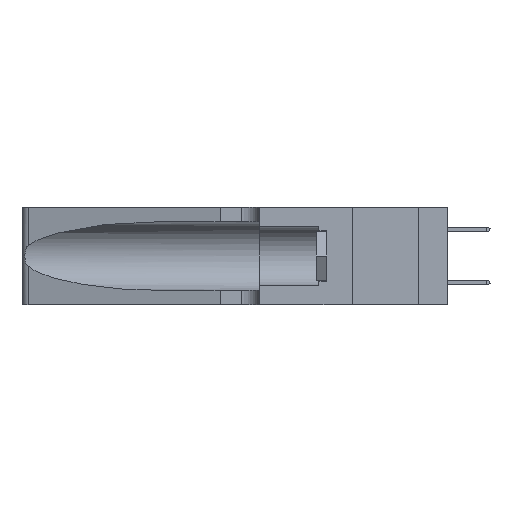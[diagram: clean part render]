
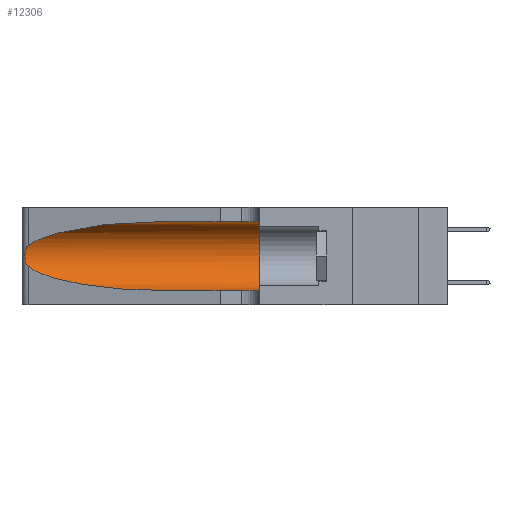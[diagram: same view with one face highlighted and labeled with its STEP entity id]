
A CAD part, left-side view. The second image highlights one B-rep face of the part: STEP entity #12306.
In plain terms, the highlighted cylindrical face has radius 3.308 mm (diameter 6.617 mm), a partial arc.
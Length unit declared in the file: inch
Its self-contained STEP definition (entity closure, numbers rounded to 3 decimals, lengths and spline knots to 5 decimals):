
#554 = CARTESIAN_POINT ( 'NONE',  ( 0.1305, 0.72297, 0.05475 ) ) ;
#833 =( BOUNDED_CURVE ( )  B_SPLINE_CURVE ( 3, ( #21666, #19783, #14229, #2589 ),
 .UNSPECIFIED., .F., .F. ) 
 B_SPLINE_CURVE_WITH_KNOTS ( ( 4, 4 ),
 ( 1.5708, 2.84003 ),
 .UNSPECIFIED. ) 
 CURVE ( )  GEOMETRIC_REPRESENTATION_ITEM ( )  RATIONAL_B_SPLINE_CURVE ( ( 1., 0.87, 0.87, 1. ) ) 
 REPRESENTATION_ITEM ( '' )  );
#1058 = CARTESIAN_POINT ( 'NONE',  ( 0.26075, 1.23896, 0.19203 ) ) ;
#1847 = CIRCLE ( 'NONE', #7283, 0.13025 ) ;
#2323 = VERTEX_POINT ( 'NONE', #22062 ) ;
#2327 = DIRECTION ( 'NONE',  ( 0., 1., 0. ) ) ;
#2589 = CARTESIAN_POINT ( 'NONE',  ( 0.25487, 1.22718, 0.22369 ) ) ;
#3119 = CARTESIAN_POINT ( 'NONE',  ( 0.26017, 1.23833, 0.17102 ) ) ;
#3168 = VERTEX_POINT ( 'NONE', #9739 ) ;
#3367 = ORIENTED_EDGE ( 'NONE', *, *, #22106, .T. ) ;
#3416 = CARTESIAN_POINT ( 'NONE',  ( 0.18966, 0.96281, 0.05475 ) ) ;
#4304 = ORIENTED_EDGE ( 'NONE', *, *, #17863, .F. ) ;
#4429 = CYLINDRICAL_SURFACE ( 'NONE', #19527, 0.13025 ) ;
#4578 =( BOUNDED_CURVE ( )  B_SPLINE_CURVE ( 3, ( #13120, #24311, #3416, #16892 ),
 .UNSPECIFIED., .F., .F. ) 
 B_SPLINE_CURVE_WITH_KNOTS ( ( 4, 4 ),
 ( 3.44316, 4.71239 ),
 .UNSPECIFIED. ) 
 CURVE ( )  GEOMETRIC_REPRESENTATION_ITEM ( )  RATIONAL_B_SPLINE_CURVE ( ( 1., 0.87, 0.87, 1. ) ) 
 REPRESENTATION_ITEM ( '' )  );
#4581 = B_SPLINE_CURVE_WITH_KNOTS ( 'NONE', 3,
 ( #12762, #9028, #22150, #10945, #24037, #12842, #1058, #14730, #3119, #16616, #5151, #18475, #7165, #20344 ),
 .UNSPECIFIED., .F., .F.,
 ( 4, 2, 2, 2, 2, 2, 4 ),
 ( 0., 0.00027, 0.00053, 0.00107, 0.0016, 0.00187, 0.00214 ),
 .UNSPECIFIED. ) ;
#5151 = CARTESIAN_POINT ( 'NONE',  ( 0.25789, 1.23486, 0.15765 ) ) ;
#6310 = EDGE_CURVE ( 'NONE', #8573, #9036, #4581, .T. ) ;
#7165 = CARTESIAN_POINT ( 'NONE',  ( 0.25555, 1.22993, 0.14849 ) ) ;
#7283 = AXIS2_PLACEMENT_3D ( 'NONE', #13997, #2327, #15899 ) ;
#8015 = CARTESIAN_POINT ( 'NONE',  ( 0.25487, 1.22718, 0.14631 ) ) ;
#8573 = VERTEX_POINT ( 'NONE', #17609 ) ;
#8667 = ORIENTED_EDGE ( 'NONE', *, *, #20192, .T. ) ;
#9028 = CARTESIAN_POINT ( 'NONE',  ( 0.25555, 1.22994, 0.2215 ) ) ;
#9036 = VERTEX_POINT ( 'NONE', #8015 ) ;
#9594 = EDGE_CURVE ( 'NONE', #23305, #2323, #19759, .T. ) ;
#9669 = FACE_OUTER_BOUND ( 'NONE', #20645, .T. ) ;
#9739 = CARTESIAN_POINT ( 'NONE',  ( 0.1305, 0.35, 0.05475 ) ) ;
#10945 = CARTESIAN_POINT ( 'NONE',  ( 0.25787, 1.23484, 0.2124 ) ) ;
#11216 = ORIENTED_EDGE ( 'NONE', *, *, #6310, .T. ) ;
#12306 = ADVANCED_FACE ( 'NONE', ( #9669 ), #4429, .F. ) ;
#12496 = VERTEX_POINT ( 'NONE', #554 ) ;
#12762 = CARTESIAN_POINT ( 'NONE',  ( 0.25487, 1.22718, 0.22369 ) ) ;
#12842 = CARTESIAN_POINT ( 'NONE',  ( 0.26018, 1.23835, 0.19895 ) ) ;
#13120 = CARTESIAN_POINT ( 'NONE',  ( 0.25487, 1.22718, 0.14631 ) ) ;
#13997 = CARTESIAN_POINT ( 'NONE',  ( 0.1305, 0.35, 0.185 ) ) ;
#14229 = CARTESIAN_POINT ( 'NONE',  ( 0.2373, 1.15595, 0.28018 ) ) ;
#14730 = CARTESIAN_POINT ( 'NONE',  ( 0.26075, 1.23896, 0.178 ) ) ;
#14997 = EDGE_CURVE ( 'NONE', #23305, #8573, #833, .T. ) ;
#15224 = DIRECTION ( 'NONE',  ( 0., -1., 0. ) ) ;
#15517 = CARTESIAN_POINT ( 'NONE',  ( 0.1305, 1.61858, 0.185 ) ) ;
#15899 = DIRECTION ( 'NONE',  ( 0., 0., 1. ) ) ;
#16616 = CARTESIAN_POINT ( 'NONE',  ( 0.25856, 1.23593, 0.16098 ) ) ;
#16892 = CARTESIAN_POINT ( 'NONE',  ( 0.1305, 0.72297, 0.05475 ) ) ;
#17609 = CARTESIAN_POINT ( 'NONE',  ( 0.25487, 1.22718, 0.22369 ) ) ;
#17810 = VECTOR ( 'NONE', #24400, 39.37008 ) ;
#17863 = EDGE_CURVE ( 'NONE', #2323, #3168, #1847, .T. ) ;
#18276 = ORIENTED_EDGE ( 'NONE', *, *, #14997, .T. ) ;
#18405 = LINE ( 'NONE', #22515, #17810 ) ;
#18475 = CARTESIAN_POINT ( 'NONE',  ( 0.25639, 1.23186, 0.15144 ) ) ;
#18962 = ORIENTED_EDGE ( 'NONE', *, *, #9594, .F. ) ;
#19527 = AXIS2_PLACEMENT_3D ( 'NONE', #15517, #21143, #23007 ) ;
#19759 = LINE ( 'NONE', #20832, #24149 ) ;
#19783 = CARTESIAN_POINT ( 'NONE',  ( 0.18966, 0.96281, 0.31525 ) ) ;
#20192 = EDGE_CURVE ( 'NONE', #9036, #12496, #4578, .T. ) ;
#20344 = CARTESIAN_POINT ( 'NONE',  ( 0.25487, 1.22718, 0.14631 ) ) ;
#20645 = EDGE_LOOP ( 'NONE', ( #18276, #11216, #8667, #3367, #4304, #18962 ) ) ;
#20832 = CARTESIAN_POINT ( 'NONE',  ( 0.1305, 1.61858, 0.31525 ) ) ;
#20865 = CARTESIAN_POINT ( 'NONE',  ( 0.1305, 0.72297, 0.31525 ) ) ;
#21143 = DIRECTION ( 'NONE',  ( 0., -1., 0. ) ) ;
#21666 = CARTESIAN_POINT ( 'NONE',  ( 0.1305, 0.72297, 0.31525 ) ) ;
#22062 = CARTESIAN_POINT ( 'NONE',  ( 0.1305, 0.35, 0.31525 ) ) ;
#22106 = EDGE_CURVE ( 'NONE', #12496, #3168, #18405, .T. ) ;
#22150 = CARTESIAN_POINT ( 'NONE',  ( 0.25639, 1.23184, 0.21858 ) ) ;
#22515 = CARTESIAN_POINT ( 'NONE',  ( 0.1305, 1.61858, 0.05475 ) ) ;
#23007 = DIRECTION ( 'NONE',  ( 0., 0., -1. ) ) ;
#23305 = VERTEX_POINT ( 'NONE', #20865 ) ;
#24037 = CARTESIAN_POINT ( 'NONE',  ( 0.25854, 1.2359, 0.20912 ) ) ;
#24149 = VECTOR ( 'NONE', #15224, 39.37008 ) ;
#24311 = CARTESIAN_POINT ( 'NONE',  ( 0.2373, 1.15595, 0.08982 ) ) ;
#24400 = DIRECTION ( 'NONE',  ( 0., -1., 0. ) ) ;
